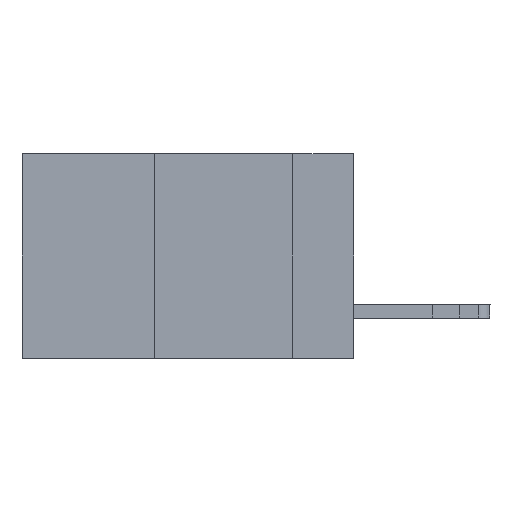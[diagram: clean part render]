
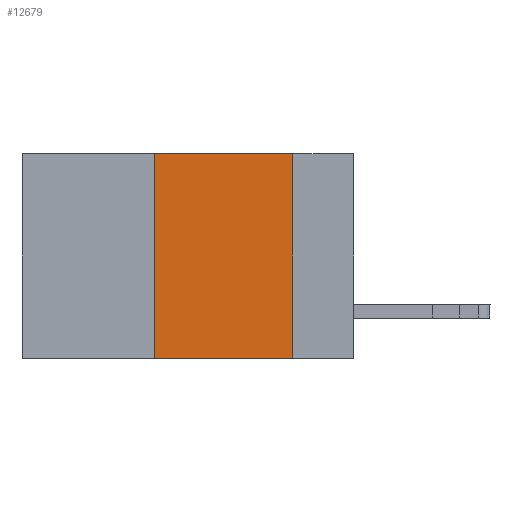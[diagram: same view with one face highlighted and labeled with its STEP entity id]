
A CAD part, left-side view. The second image highlights one B-rep face of the part: STEP entity #12679.
In plain terms, the highlighted planar face has unit normal (-1, 0, 0).
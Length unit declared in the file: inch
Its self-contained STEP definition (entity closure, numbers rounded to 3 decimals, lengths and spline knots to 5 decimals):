
#26 = ORIENTED_EDGE ( 'NONE', *, *, #14301, .T. ) ;
#227 = ORIENTED_EDGE ( 'NONE', *, *, #12469, .F. ) ;
#966 = VECTOR ( 'NONE', #12374, 39.37008 ) ;
#2365 = CARTESIAN_POINT ( 'NONE',  ( 0., 0.36, -0.37 ) ) ;
#2920 = EDGE_CURVE ( 'NONE', #13229, #10928, #6439, .T. ) ;
#2996 = ORIENTED_EDGE ( 'NONE', *, *, #8327, .F. ) ;
#3291 = VECTOR ( 'NONE', #10123, 39.37008 ) ;
#4231 = CARTESIAN_POINT ( 'NONE',  ( 0., 0.11, -0.37 ) ) ;
#4418 = LINE ( 'NONE', #6084, #966 ) ;
#4436 = DIRECTION ( 'NONE',  ( 0., -1., 0. ) ) ;
#5621 = PLANE ( 'NONE',  #16324 ) ;
#5680 = DIRECTION ( 'NONE',  ( 0., 0., -1. ) ) ;
#5742 = LINE ( 'NONE', #15110, #6969 ) ;
#5909 = CARTESIAN_POINT ( 'NONE',  ( 0., 0.11, 0. ) ) ;
#5965 = ORIENTED_EDGE ( 'NONE', *, *, #2920, .F. ) ;
#6084 = CARTESIAN_POINT ( 'NONE',  ( 0., 0.6, -0.37 ) ) ;
#6439 = LINE ( 'NONE', #15712, #14108 ) ;
#6752 = LINE ( 'NONE', #10301, #3291 ) ;
#6969 = VECTOR ( 'NONE', #7374, 39.37008 ) ;
#7374 = DIRECTION ( 'NONE',  ( 0., 0., -1. ) ) ;
#8327 = EDGE_CURVE ( 'NONE', #10928, #14614, #5742, .T. ) ;
#10123 = DIRECTION ( 'NONE',  ( 0., 0., 1. ) ) ;
#10197 = FACE_OUTER_BOUND ( 'NONE', #16297, .T. ) ;
#10301 = CARTESIAN_POINT ( 'NONE',  ( 0., 0.36, 0. ) ) ;
#10928 = VERTEX_POINT ( 'NONE', #5909 ) ;
#12374 = DIRECTION ( 'NONE',  ( 0., -1., 0. ) ) ;
#12469 = EDGE_CURVE ( 'NONE', #13046, #13229, #6752, .T. ) ;
#12679 = ADVANCED_FACE ( 'NONE', ( #10197 ), #5621, .F. ) ;
#13046 = VERTEX_POINT ( 'NONE', #2365 ) ;
#13229 = VERTEX_POINT ( 'NONE', #14247 ) ;
#14108 = VECTOR ( 'NONE', #4436, 39.37008 ) ;
#14247 = CARTESIAN_POINT ( 'NONE',  ( 0., 0.36, 0. ) ) ;
#14301 = EDGE_CURVE ( 'NONE', #13046, #14614, #4418, .T. ) ;
#14614 = VERTEX_POINT ( 'NONE', #4231 ) ;
#14698 = CARTESIAN_POINT ( 'NONE',  ( 0., 0.6, 0. ) ) ;
#15110 = CARTESIAN_POINT ( 'NONE',  ( 0., 0.11, 0. ) ) ;
#15712 = CARTESIAN_POINT ( 'NONE',  ( 0., 0.6, 0. ) ) ;
#15967 = DIRECTION ( 'NONE',  ( 1., 0., 0. ) ) ;
#16297 = EDGE_LOOP ( 'NONE', ( #2996, #5965, #227, #26 ) ) ;
#16324 = AXIS2_PLACEMENT_3D ( 'NONE', #14698, #15967, #5680 ) ;
